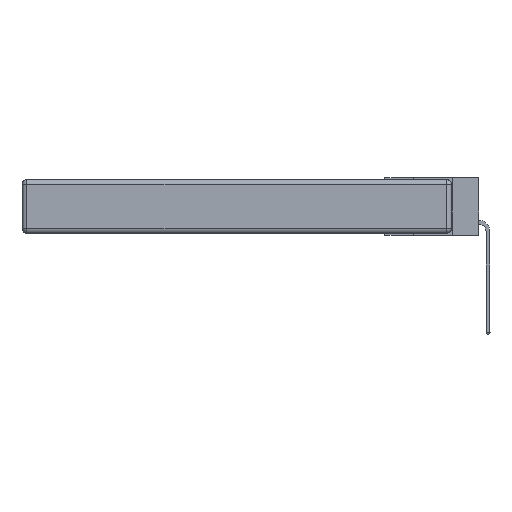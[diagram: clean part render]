
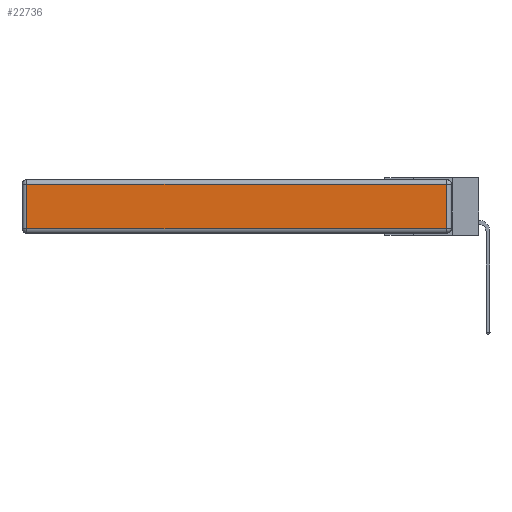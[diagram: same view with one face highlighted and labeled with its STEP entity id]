
A CAD part, left-side view. The second image highlights one B-rep face of the part: STEP entity #22736.
In plain terms, the highlighted planar face has unit normal (-1, 0, 0).
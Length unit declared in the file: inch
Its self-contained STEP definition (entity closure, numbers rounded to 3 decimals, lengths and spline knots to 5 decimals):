
#725 = ORIENTED_EDGE ( 'NONE', *, *, #8175, .T. ) ;
#1682 = DIRECTION ( 'NONE',  ( -1., 0., 0. ) ) ;
#2001 = DIRECTION ( 'NONE',  ( 0., 1., 0. ) ) ;
#2346 = AXIS2_PLACEMENT_3D ( 'NONE', #9136, #1682, #17001 ) ;
#2921 = LINE ( 'NONE', #9705, #22865 ) ;
#3452 = PLANE ( 'NONE',  #2346 ) ;
#3562 = EDGE_LOOP ( 'NONE', ( #5781, #725, #5519, #13329 ) ) ;
#5096 = DIRECTION ( 'NONE',  ( 0., 0., -1. ) ) ;
#5519 = ORIENTED_EDGE ( 'NONE', *, *, #18857, .T. ) ;
#5781 = ORIENTED_EDGE ( 'NONE', *, *, #17824, .T. ) ;
#5818 = CARTESIAN_POINT ( 'NONE',  ( 0., 0.03, -0.313 ) ) ;
#7429 = LINE ( 'NONE', #8263, #24630 ) ;
#8175 = EDGE_CURVE ( 'NONE', #22864, #24446, #7429, .T. ) ;
#8263 = CARTESIAN_POINT ( 'NONE',  ( 0., 0.03, -0.343 ) ) ;
#8490 = LINE ( 'NONE', #14585, #19025 ) ;
#9136 = CARTESIAN_POINT ( 'NONE',  ( 0., 0., -0.343 ) ) ;
#9532 = CARTESIAN_POINT ( 'NONE',  ( 0., 2.72, -0.03 ) ) ;
#9705 = CARTESIAN_POINT ( 'NONE',  ( 0., 2.75, -0.03 ) ) ;
#10331 = VERTEX_POINT ( 'NONE', #9532 ) ;
#11140 = FACE_OUTER_BOUND ( 'NONE', #3562, .T. ) ;
#13329 = ORIENTED_EDGE ( 'NONE', *, *, #21079, .T. ) ;
#14427 = VERTEX_POINT ( 'NONE', #17229 ) ;
#14585 = CARTESIAN_POINT ( 'NONE',  ( 0., 2.72, -0.343 ) ) ;
#17001 = DIRECTION ( 'NONE',  ( 0., 0., 1. ) ) ;
#17174 = LINE ( 'NONE', #23176, #21979 ) ;
#17229 = CARTESIAN_POINT ( 'NONE',  ( 0., 2.72, -0.313 ) ) ;
#17384 = DIRECTION ( 'NONE',  ( 0., -1., 0. ) ) ;
#17550 = CARTESIAN_POINT ( 'NONE',  ( 0., 0.03, -0.03 ) ) ;
#17824 = EDGE_CURVE ( 'NONE', #14427, #22864, #17174, .T. ) ;
#18857 = EDGE_CURVE ( 'NONE', #24446, #10331, #2921, .T. ) ;
#19025 = VECTOR ( 'NONE', #5096, 39.37008 ) ;
#21079 = EDGE_CURVE ( 'NONE', #10331, #14427, #8490, .T. ) ;
#21772 = DIRECTION ( 'NONE',  ( 0., 0., 1. ) ) ;
#21979 = VECTOR ( 'NONE', #17384, 39.37008 ) ;
#22736 = ADVANCED_FACE ( 'NONE', ( #11140 ), #3452, .T. ) ;
#22864 = VERTEX_POINT ( 'NONE', #5818 ) ;
#22865 = VECTOR ( 'NONE', #2001, 39.37008 ) ;
#23176 = CARTESIAN_POINT ( 'NONE',  ( 0., 0., -0.313 ) ) ;
#24446 = VERTEX_POINT ( 'NONE', #17550 ) ;
#24630 = VECTOR ( 'NONE', #21772, 39.37008 ) ;
